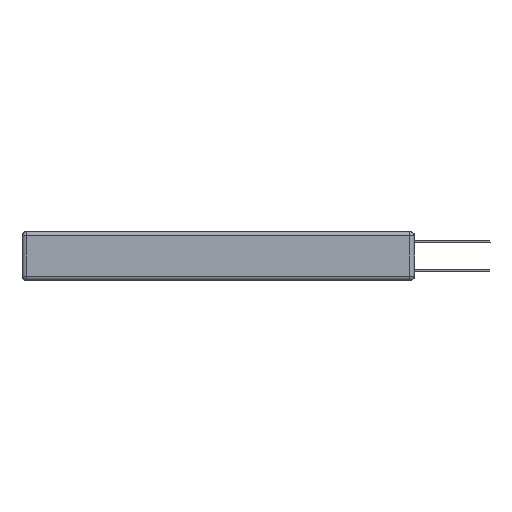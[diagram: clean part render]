
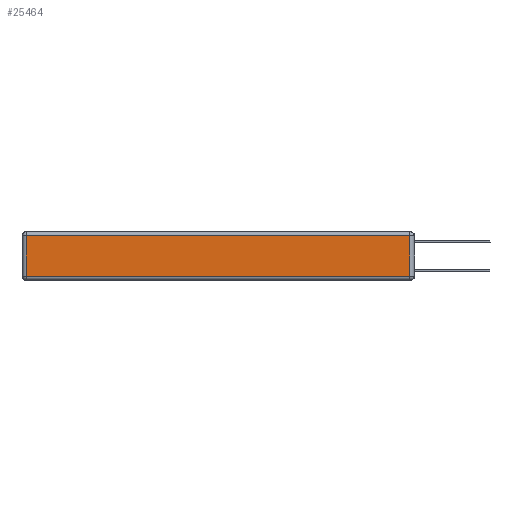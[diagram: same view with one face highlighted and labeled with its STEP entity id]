
A CAD part, left-side view. The second image highlights one B-rep face of the part: STEP entity #25464.
In plain terms, the highlighted planar face has unit normal (-1, 0, 0).
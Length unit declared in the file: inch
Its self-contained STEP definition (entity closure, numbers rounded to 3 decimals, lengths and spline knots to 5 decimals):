
#485 = VERTEX_POINT ( 'NONE', #18590 ) ;
#980 = VERTEX_POINT ( 'NONE', #6094 ) ;
#1252 = DIRECTION ( 'NONE',  ( -1., 0., 0. ) ) ;
#2451 = ORIENTED_EDGE ( 'NONE', *, *, #3735, .T. ) ;
#3037 = LINE ( 'NONE', #20574, #10997 ) ;
#3735 = EDGE_CURVE ( 'NONE', #24682, #23782, #3037, .T. ) ;
#4247 = CARTESIAN_POINT ( 'NONE',  ( 0., 2.72, -0.343 ) ) ;
#5444 = VECTOR ( 'NONE', #22652, 39.37008 ) ;
#6094 = CARTESIAN_POINT ( 'NONE',  ( 0., 2.72, -0.313 ) ) ;
#7673 = VECTOR ( 'NONE', #15827, 39.37008 ) ;
#8913 = CARTESIAN_POINT ( 'NONE',  ( 0., 0.03, -0.03 ) ) ;
#9416 = PLANE ( 'NONE',  #19934 ) ;
#10452 = DIRECTION ( 'NONE',  ( 0., 0., 1. ) ) ;
#10846 = LINE ( 'NONE', #24693, #5444 ) ;
#10997 = VECTOR ( 'NONE', #10452, 39.37008 ) ;
#12080 = LINE ( 'NONE', #4247, #20965 ) ;
#13488 = CARTESIAN_POINT ( 'NONE',  ( 0., 0., -0.343 ) ) ;
#14283 = DIRECTION ( 'NONE',  ( 0., 0., -1. ) ) ;
#15406 = ORIENTED_EDGE ( 'NONE', *, *, #25113, .T. ) ;
#15827 = DIRECTION ( 'NONE',  ( 0., 1., 0. ) ) ;
#16462 = CARTESIAN_POINT ( 'NONE',  ( 0., 0.03, -0.313 ) ) ;
#16564 = LINE ( 'NONE', #25675, #7673 ) ;
#18590 = CARTESIAN_POINT ( 'NONE',  ( 0., 2.72, -0.03 ) ) ;
#18788 = FACE_OUTER_BOUND ( 'NONE', #23315, .T. ) ;
#18884 = ORIENTED_EDGE ( 'NONE', *, *, #25309, .T. ) ;
#19934 = AXIS2_PLACEMENT_3D ( 'NONE', #13488, #1252, #22917 ) ;
#20574 = CARTESIAN_POINT ( 'NONE',  ( 0., 0.03, -0.343 ) ) ;
#20965 = VECTOR ( 'NONE', #14283, 39.37008 ) ;
#21636 = ORIENTED_EDGE ( 'NONE', *, *, #25823, .T. ) ;
#22652 = DIRECTION ( 'NONE',  ( 0., -1., 0. ) ) ;
#22917 = DIRECTION ( 'NONE',  ( 0., 0., 1. ) ) ;
#23315 = EDGE_LOOP ( 'NONE', ( #18884, #2451, #15406, #21636 ) ) ;
#23782 = VERTEX_POINT ( 'NONE', #8913 ) ;
#24682 = VERTEX_POINT ( 'NONE', #16462 ) ;
#24693 = CARTESIAN_POINT ( 'NONE',  ( 0., 0., -0.313 ) ) ;
#25113 = EDGE_CURVE ( 'NONE', #23782, #485, #16564, .T. ) ;
#25309 = EDGE_CURVE ( 'NONE', #980, #24682, #10846, .T. ) ;
#25464 = ADVANCED_FACE ( 'NONE', ( #18788 ), #9416, .T. ) ;
#25675 = CARTESIAN_POINT ( 'NONE',  ( 0., 2.75, -0.03 ) ) ;
#25823 = EDGE_CURVE ( 'NONE', #485, #980, #12080, .T. ) ;
